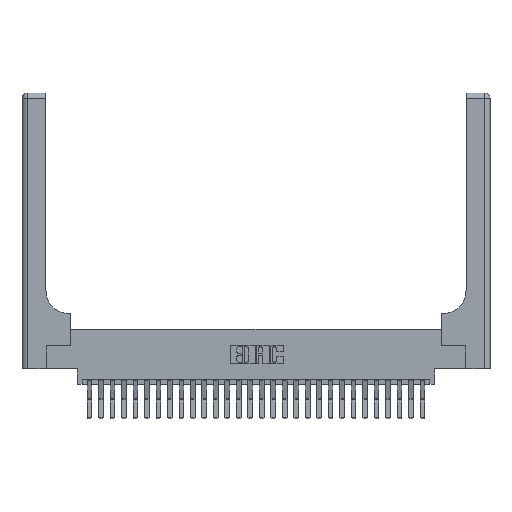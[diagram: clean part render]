
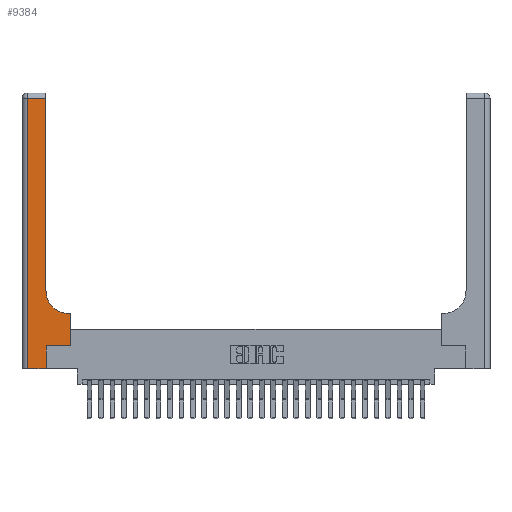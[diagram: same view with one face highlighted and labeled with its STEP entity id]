
A CAD part, top view. The second image highlights one B-rep face of the part: STEP entity #9384.
In plain terms, the highlighted planar face has unit normal (0, 0, 1).
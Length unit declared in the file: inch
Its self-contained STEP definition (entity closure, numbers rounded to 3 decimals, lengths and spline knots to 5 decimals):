
#38 = VERTEX_POINT ( 'NONE', #10832 ) ;
#159 = LINE ( 'NONE', #23052, #10070 ) ;
#1094 = DIRECTION ( 'NONE',  ( 0., 1., 0. ) ) ;
#1169 = VECTOR ( 'NONE', #19772, 39.37008 ) ;
#1339 = CARTESIAN_POINT ( 'NONE',  ( 0.06, 3., 0.37 ) ) ;
#1932 = ORIENTED_EDGE ( 'NONE', *, *, #3735, .T. ) ;
#1976 = DIRECTION ( 'NONE',  ( 1., 0., 0. ) ) ;
#2007 = DIRECTION ( 'NONE',  ( -1., 0., 0. ) ) ;
#2146 = CARTESIAN_POINT ( 'NONE',  ( 0.26, 0.6, 0.37 ) ) ;
#2963 = ORIENTED_EDGE ( 'NONE', *, *, #4679, .T. ) ;
#3080 = LINE ( 'NONE', #11431, #1169 ) ;
#3484 = PLANE ( 'NONE',  #24568 ) ;
#3553 = ORIENTED_EDGE ( 'NONE', *, *, #21587, .T. ) ;
#3735 = EDGE_CURVE ( 'NONE', #11307, #9529, #159, .T. ) ;
#4679 = EDGE_CURVE ( 'NONE', #20144, #38, #14350, .T. ) ;
#4826 = VERTEX_POINT ( 'NONE', #20187 ) ;
#5039 = VERTEX_POINT ( 'NONE', #24727 ) ;
#5112 = VECTOR ( 'NONE', #2007, 39.37008 ) ;
#5272 = ORIENTED_EDGE ( 'NONE', *, *, #22120, .T. ) ;
#5670 = EDGE_CURVE ( 'NONE', #17156, #11307, #15715, .T. ) ;
#5932 = EDGE_CURVE ( 'NONE', #11474, #5039, #9003, .T. ) ;
#6484 = AXIS2_PLACEMENT_3D ( 'NONE', #17143, #23071, #1976 ) ;
#7064 = EDGE_CURVE ( 'NONE', #9529, #20144, #11634, .T. ) ;
#7409 = CARTESIAN_POINT ( 'NONE',  ( 0.06, 2.94, 0.37 ) ) ;
#7446 = ORIENTED_EDGE ( 'NONE', *, *, #7064, .T. ) ;
#8820 = CARTESIAN_POINT ( 'NONE',  ( 0.265, 0.25, 0.37 ) ) ;
#9003 = LINE ( 'NONE', #17200, #18478 ) ;
#9384 = ADVANCED_FACE ( 'NONE', ( #18137 ), #3484, .F. ) ;
#9529 = VERTEX_POINT ( 'NONE', #22791 ) ;
#9660 = VERTEX_POINT ( 'NONE', #17954 ) ;
#9861 = VECTOR ( 'NONE', #26382, 39.37008 ) ;
#10070 = VECTOR ( 'NONE', #14823, 39.37008 ) ;
#10241 = CARTESIAN_POINT ( 'NONE',  ( 0.265, 0.25, 0.37 ) ) ;
#10364 = LINE ( 'NONE', #16775, #17825 ) ;
#10832 = CARTESIAN_POINT ( 'NONE',  ( 0.528, 0.25, 0.37 ) ) ;
#11307 = VERTEX_POINT ( 'NONE', #22793 ) ;
#11431 = CARTESIAN_POINT ( 'NONE',  ( 0., 2.94, 0.37 ) ) ;
#11474 = VERTEX_POINT ( 'NONE', #23079 ) ;
#11634 = LINE ( 'NONE', #19711, #23380 ) ;
#12116 = ORIENTED_EDGE ( 'NONE', *, *, #21823, .T. ) ;
#12796 = LINE ( 'NONE', #2146, #5112 ) ;
#13152 = ORIENTED_EDGE ( 'NONE', *, *, #5670, .T. ) ;
#14350 = LINE ( 'NONE', #10241, #24264 ) ;
#14823 = DIRECTION ( 'NONE',  ( 1., 0., 0. ) ) ;
#15539 = EDGE_LOOP ( 'NONE', ( #26551, #12116, #13152, #1932, #7446, #2963, #3553, #21437, #5272 ) ) ;
#15715 = LINE ( 'NONE', #1339, #9861 ) ;
#16775 = CARTESIAN_POINT ( 'NONE',  ( 0.528, 0.25, 0.37 ) ) ;
#17143 = CARTESIAN_POINT ( 'NONE',  ( 0.51, 0.85, 0.37 ) ) ;
#17156 = VERTEX_POINT ( 'NONE', #7409 ) ;
#17200 = CARTESIAN_POINT ( 'NONE',  ( 0.26, 3., 0.37 ) ) ;
#17388 = DIRECTION ( 'NONE',  ( 0., 1., 0. ) ) ;
#17825 = VECTOR ( 'NONE', #17388, 39.37008 ) ;
#17859 = CARTESIAN_POINT ( 'NONE',  ( 0., 3., 0.37 ) ) ;
#17954 = CARTESIAN_POINT ( 'NONE',  ( 0.528, 0.6, 0.37 ) ) ;
#18137 = FACE_OUTER_BOUND ( 'NONE', #15539, .T. ) ;
#18400 = DIRECTION ( 'NONE',  ( -1., 0., 0. ) ) ;
#18478 = VECTOR ( 'NONE', #25577, 39.37008 ) ;
#18593 = DIRECTION ( 'NONE',  ( 1., 0., 0. ) ) ;
#19711 = CARTESIAN_POINT ( 'NONE',  ( 0.265, 0., 0.37 ) ) ;
#19772 = DIRECTION ( 'NONE',  ( -1., 0., 0. ) ) ;
#20144 = VERTEX_POINT ( 'NONE', #8820 ) ;
#20187 = CARTESIAN_POINT ( 'NONE',  ( 0.51, 0.6, 0.37 ) ) ;
#20208 = EDGE_CURVE ( 'NONE', #9660, #4826, #12796, .T. ) ;
#21437 = ORIENTED_EDGE ( 'NONE', *, *, #20208, .T. ) ;
#21587 = EDGE_CURVE ( 'NONE', #38, #9660, #10364, .T. ) ;
#21728 = CIRCLE ( 'NONE', #6484, 0.25 ) ;
#21823 = EDGE_CURVE ( 'NONE', #5039, #17156, #3080, .T. ) ;
#22120 = EDGE_CURVE ( 'NONE', #4826, #11474, #21728, .T. ) ;
#22791 = CARTESIAN_POINT ( 'NONE',  ( 0.265, 0., 0.37 ) ) ;
#22793 = CARTESIAN_POINT ( 'NONE',  ( 0.06, 0., 0.37 ) ) ;
#23052 = CARTESIAN_POINT ( 'NONE',  ( 0., 0., 0.37 ) ) ;
#23071 = DIRECTION ( 'NONE',  ( 0., 0., -1. ) ) ;
#23079 = CARTESIAN_POINT ( 'NONE',  ( 0.26, 0.85, 0.37 ) ) ;
#23380 = VECTOR ( 'NONE', #1094, 39.37008 ) ;
#24159 = DIRECTION ( 'NONE',  ( 0., 0., -1. ) ) ;
#24264 = VECTOR ( 'NONE', #18593, 39.37008 ) ;
#24568 = AXIS2_PLACEMENT_3D ( 'NONE', #17859, #24159, #18400 ) ;
#24727 = CARTESIAN_POINT ( 'NONE',  ( 0.26, 2.94, 0.37 ) ) ;
#25577 = DIRECTION ( 'NONE',  ( 0., 1., 0. ) ) ;
#26382 = DIRECTION ( 'NONE',  ( 0., -1., 0. ) ) ;
#26551 = ORIENTED_EDGE ( 'NONE', *, *, #5932, .T. ) ;
